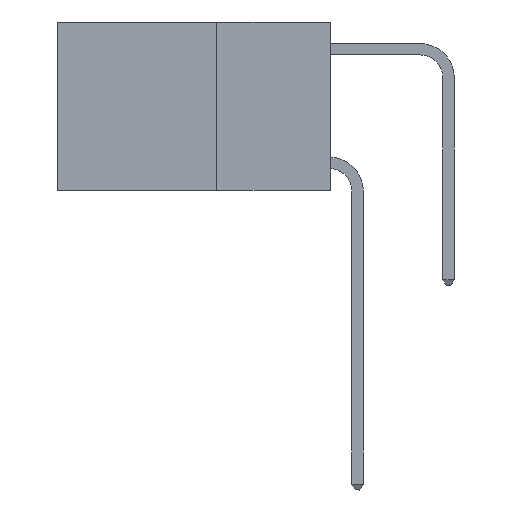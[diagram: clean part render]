
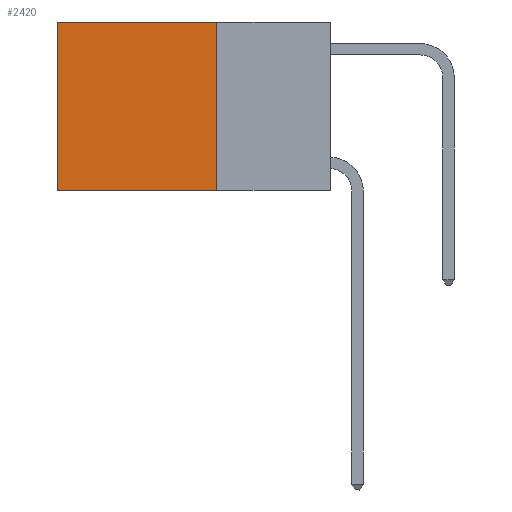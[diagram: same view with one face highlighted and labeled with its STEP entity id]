
A CAD part, left-side view. The second image highlights one B-rep face of the part: STEP entity #2420.
In plain terms, the highlighted planar face has unit normal (-1, 0, 0).
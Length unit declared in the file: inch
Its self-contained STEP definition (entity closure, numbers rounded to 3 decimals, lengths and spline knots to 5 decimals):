
#461 = CARTESIAN_POINT ( 'NONE',  ( 0.2625, 0.6, 0. ) ) ;
#1328 = FACE_OUTER_BOUND ( 'NONE', #11963, .T. ) ;
#1495 = VECTOR ( 'NONE', #9116, 39.37008 ) ;
#2420 = ADVANCED_FACE ( 'NONE', ( #1328 ), #10195, .F. ) ;
#2434 = LINE ( 'NONE', #11126, #7105 ) ;
#2802 = CARTESIAN_POINT ( 'NONE',  ( 0.2625, 0.25, -0.37 ) ) ;
#3371 = EDGE_CURVE ( 'NONE', #5750, #13932, #7787, .T. ) ;
#3640 = CARTESIAN_POINT ( 'NONE',  ( 0.2625, 0.25, -0.37 ) ) ;
#3923 = ORIENTED_EDGE ( 'NONE', *, *, #3371, .T. ) ;
#4204 = LINE ( 'NONE', #12759, #1495 ) ;
#4739 = VECTOR ( 'NONE', #7820, 39.37008 ) ;
#5750 = VERTEX_POINT ( 'NONE', #15817 ) ;
#6937 = EDGE_CURVE ( 'NONE', #14466, #14536, #2434, .T. ) ;
#7067 = ORIENTED_EDGE ( 'NONE', *, *, #9385, .T. ) ;
#7105 = VECTOR ( 'NONE', #13455, 39.37008 ) ;
#7787 = LINE ( 'NONE', #461, #10626 ) ;
#7820 = DIRECTION ( 'NONE',  ( 0., 1., 0. ) ) ;
#8672 = AXIS2_PLACEMENT_3D ( 'NONE', #15087, #10031, #13373 ) ;
#9116 = DIRECTION ( 'NONE',  ( 0., 1., 0. ) ) ;
#9385 = EDGE_CURVE ( 'NONE', #14466, #5750, #4204, .T. ) ;
#10031 = DIRECTION ( 'NONE',  ( 1., 0., 0. ) ) ;
#10195 = PLANE ( 'NONE',  #8672 ) ;
#10626 = VECTOR ( 'NONE', #14116, 39.37008 ) ;
#10722 = CARTESIAN_POINT ( 'NONE',  ( 0.2625, 0.6, -0.37 ) ) ;
#10846 = CARTESIAN_POINT ( 'NONE',  ( 0.2625, 0.25, 0. ) ) ;
#11065 = ORIENTED_EDGE ( 'NONE', *, *, #12108, .F. ) ;
#11126 = CARTESIAN_POINT ( 'NONE',  ( 0.2625, 0.25, 0. ) ) ;
#11329 = ORIENTED_EDGE ( 'NONE', *, *, #6937, .F. ) ;
#11963 = EDGE_LOOP ( 'NONE', ( #3923, #11065, #11329, #7067 ) ) ;
#12108 = EDGE_CURVE ( 'NONE', #14536, #13932, #13996, .T. ) ;
#12759 = CARTESIAN_POINT ( 'NONE',  ( 0.2625, 0.25, 0. ) ) ;
#13373 = DIRECTION ( 'NONE',  ( 0., 0., -1. ) ) ;
#13455 = DIRECTION ( 'NONE',  ( 0., 0., -1. ) ) ;
#13932 = VERTEX_POINT ( 'NONE', #10722 ) ;
#13996 = LINE ( 'NONE', #2802, #4739 ) ;
#14116 = DIRECTION ( 'NONE',  ( 0., 0., -1. ) ) ;
#14466 = VERTEX_POINT ( 'NONE', #10846 ) ;
#14536 = VERTEX_POINT ( 'NONE', #3640 ) ;
#15087 = CARTESIAN_POINT ( 'NONE',  ( 0.2625, 0.25, 0. ) ) ;
#15817 = CARTESIAN_POINT ( 'NONE',  ( 0.2625, 0.6, 0. ) ) ;
